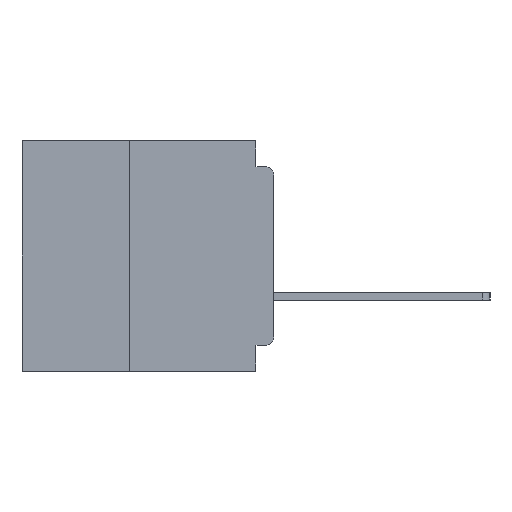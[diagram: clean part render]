
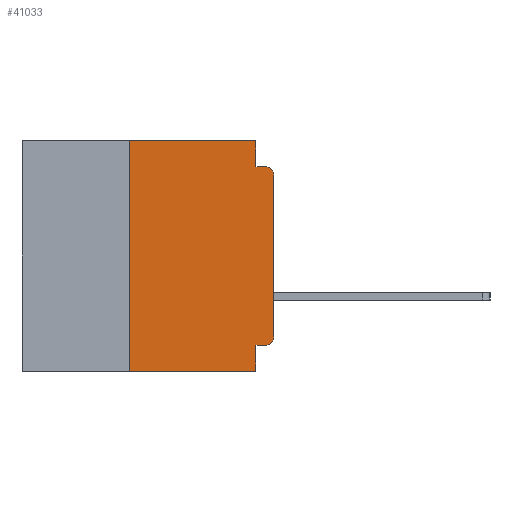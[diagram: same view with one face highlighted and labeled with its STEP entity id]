
A CAD part, left-side view. The second image highlights one B-rep face of the part: STEP entity #41033.
In plain terms, the highlighted planar face has unit normal (-1, 0, 0).
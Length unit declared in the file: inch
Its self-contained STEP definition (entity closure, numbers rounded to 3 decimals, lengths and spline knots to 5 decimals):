
#192 = CARTESIAN_POINT ( 'NONE',  ( 0., 0.015, -0.34 ) ) ;
#684 = DIRECTION ( 'NONE',  ( 0., 0., -1. ) ) ;
#918 = CARTESIAN_POINT ( 'NONE',  ( 0., 0.031, -0.045 ) ) ;
#1184 = CARTESIAN_POINT ( 'NONE',  ( 0., 0.031, -0.4 ) ) ;
#1356 = LINE ( 'NONE', #14647, #14317 ) ;
#1936 = VERTEX_POINT ( 'NONE', #27411 ) ;
#2366 = CARTESIAN_POINT ( 'NONE',  ( 0., 0.25, -0.4 ) ) ;
#2794 = CARTESIAN_POINT ( 'NONE',  ( 0., 0., -0.045 ) ) ;
#3718 = EDGE_CURVE ( 'NONE', #19269, #44134, #18645, .T. ) ;
#4103 = CARTESIAN_POINT ( 'NONE',  ( 0., 0.031, 0. ) ) ;
#4449 = CARTESIAN_POINT ( 'NONE',  ( 0., 0.015, -0.045 ) ) ;
#4613 = DIRECTION ( 'NONE',  ( 0., 0., -1. ) ) ;
#7236 = DIRECTION ( 'NONE',  ( 0., -1., 0. ) ) ;
#8040 = EDGE_CURVE ( 'NONE', #10464, #33967, #20352, .T. ) ;
#8592 = CIRCLE ( 'NONE', #31206, 0.015 ) ;
#8769 = VECTOR ( 'NONE', #15913, 39.37008 ) ;
#9180 = ORIENTED_EDGE ( 'NONE', *, *, #32966, .T. ) ;
#10187 = DIRECTION ( 'NONE',  ( -1., 0., 0. ) ) ;
#10293 = VERTEX_POINT ( 'NONE', #55728 ) ;
#10464 = VERTEX_POINT ( 'NONE', #918 ) ;
#10701 = VERTEX_POINT ( 'NONE', #37297 ) ;
#11170 = ORIENTED_EDGE ( 'NONE', *, *, #45314, .F. ) ;
#12292 = VECTOR ( 'NONE', #19668, 39.37008 ) ;
#12390 = CARTESIAN_POINT ( 'NONE',  ( 0., 0.437, 0. ) ) ;
#14033 = ORIENTED_EDGE ( 'NONE', *, *, #23882, .F. ) ;
#14317 = VECTOR ( 'NONE', #44727, 39.37008 ) ;
#14647 = CARTESIAN_POINT ( 'NONE',  ( 0., 0., 0. ) ) ;
#15794 = FACE_OUTER_BOUND ( 'NONE', #30663, .T. ) ;
#15856 = ORIENTED_EDGE ( 'NONE', *, *, #3718, .T. ) ;
#15913 = DIRECTION ( 'NONE',  ( 0., -1., 0. ) ) ;
#16245 = ORIENTED_EDGE ( 'NONE', *, *, #22535, .F. ) ;
#17426 = CARTESIAN_POINT ( 'NONE',  ( 0., 0., -0.06 ) ) ;
#18645 = LINE ( 'NONE', #50182, #54169 ) ;
#19269 = VERTEX_POINT ( 'NONE', #36784 ) ;
#19668 = DIRECTION ( 'NONE',  ( 0., 0., 1. ) ) ;
#20138 = VERTEX_POINT ( 'NONE', #17426 ) ;
#20352 = LINE ( 'NONE', #2794, #8769 ) ;
#22389 = PLANE ( 'NONE',  #23798 ) ;
#22394 = LINE ( 'NONE', #12390, #33880 ) ;
#22535 = EDGE_CURVE ( 'NONE', #19269, #34263, #35329, .T. ) ;
#22878 = EDGE_CURVE ( 'NONE', #10701, #10293, #29268, .T. ) ;
#23798 = AXIS2_PLACEMENT_3D ( 'NONE', #43741, #26779, #684 ) ;
#23882 = EDGE_CURVE ( 'NONE', #46307, #10464, #50838, .T. ) ;
#24222 = ORIENTED_EDGE ( 'NONE', *, *, #22878, .T. ) ;
#25424 = VECTOR ( 'NONE', #39635, 39.37008 ) ;
#25539 = CARTESIAN_POINT ( 'NONE',  ( 0., 0.031, 0. ) ) ;
#26130 = ORIENTED_EDGE ( 'NONE', *, *, #27561, .F. ) ;
#26711 = ORIENTED_EDGE ( 'NONE', *, *, #55507, .F. ) ;
#26779 = DIRECTION ( 'NONE',  ( 1., 0., 0. ) ) ;
#27411 = CARTESIAN_POINT ( 'NONE',  ( 0., 0.031, -0.355 ) ) ;
#27561 = EDGE_CURVE ( 'NONE', #1936, #44134, #30477, .T. ) ;
#28401 = EDGE_CURVE ( 'NONE', #20138, #33967, #8592, .T. ) ;
#29127 = VECTOR ( 'NONE', #38998, 39.37008 ) ;
#29268 = CIRCLE ( 'NONE', #31382, 0.015 ) ;
#30477 = LINE ( 'NONE', #43250, #29127 ) ;
#30645 = DIRECTION ( 'NONE',  ( -1., 0., 0. ) ) ;
#30663 = EDGE_LOOP ( 'NONE', ( #9180, #36678, #54149, #14033, #26711, #16245, #15856, #26130, #11170, #24222 ) ) ;
#31206 = AXIS2_PLACEMENT_3D ( 'NONE', #36139, #10187, #40388 ) ;
#31382 = AXIS2_PLACEMENT_3D ( 'NONE', #192, #30645, #4613 ) ;
#32966 = EDGE_CURVE ( 'NONE', #10293, #20138, #1356, .T. ) ;
#33880 = VECTOR ( 'NONE', #34001, 39.37008 ) ;
#33967 = VERTEX_POINT ( 'NONE', #4449 ) ;
#34001 = DIRECTION ( 'NONE',  ( 0., -1., 0. ) ) ;
#34263 = VERTEX_POINT ( 'NONE', #46260 ) ;
#35329 = LINE ( 'NONE', #2366, #12292 ) ;
#36139 = CARTESIAN_POINT ( 'NONE',  ( 0., 0.015, -0.06 ) ) ;
#36678 = ORIENTED_EDGE ( 'NONE', *, *, #28401, .T. ) ;
#36784 = CARTESIAN_POINT ( 'NONE',  ( 0., 0.25, -0.4 ) ) ;
#37297 = CARTESIAN_POINT ( 'NONE',  ( 0., 0.015, -0.355 ) ) ;
#38187 = LINE ( 'NONE', #48222, #25424 ) ;
#38284 = DIRECTION ( 'NONE',  ( 0., 0., -1. ) ) ;
#38998 = DIRECTION ( 'NONE',  ( 0., 0., -1. ) ) ;
#39635 = DIRECTION ( 'NONE',  ( 0., 1., 0. ) ) ;
#40388 = DIRECTION ( 'NONE',  ( 0., 0., -1. ) ) ;
#40824 = VECTOR ( 'NONE', #38284, 39.37008 ) ;
#41033 = ADVANCED_FACE ( 'NONE', ( #15794 ), #22389, .F. ) ;
#43250 = CARTESIAN_POINT ( 'NONE',  ( 0., 0.031, -0.4 ) ) ;
#43741 = CARTESIAN_POINT ( 'NONE',  ( 0., 0.437, 0. ) ) ;
#44134 = VERTEX_POINT ( 'NONE', #1184 ) ;
#44727 = DIRECTION ( 'NONE',  ( 0., 0., 1. ) ) ;
#45314 = EDGE_CURVE ( 'NONE', #10701, #1936, #38187, .T. ) ;
#46260 = CARTESIAN_POINT ( 'NONE',  ( 0., 0.25, 0. ) ) ;
#46307 = VERTEX_POINT ( 'NONE', #4103 ) ;
#48222 = CARTESIAN_POINT ( 'NONE',  ( 0., 0., -0.355 ) ) ;
#50182 = CARTESIAN_POINT ( 'NONE',  ( 0., 0.437, -0.4 ) ) ;
#50838 = LINE ( 'NONE', #25539, #40824 ) ;
#54149 = ORIENTED_EDGE ( 'NONE', *, *, #8040, .F. ) ;
#54169 = VECTOR ( 'NONE', #7236, 39.37008 ) ;
#55507 = EDGE_CURVE ( 'NONE', #34263, #46307, #22394, .T. ) ;
#55728 = CARTESIAN_POINT ( 'NONE',  ( 0., 0., -0.34 ) ) ;
